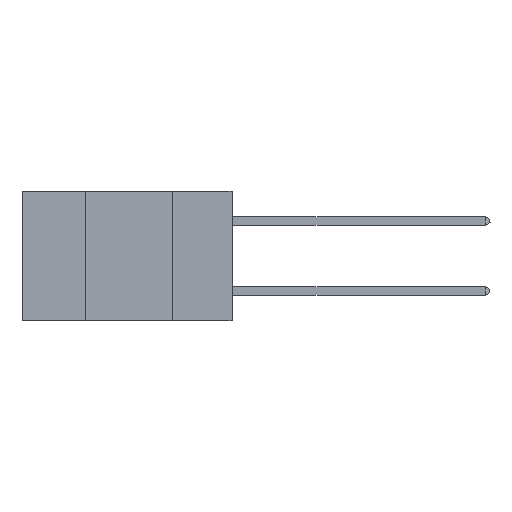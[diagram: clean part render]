
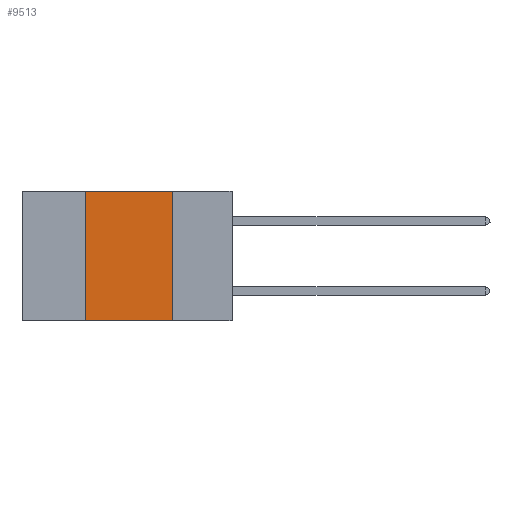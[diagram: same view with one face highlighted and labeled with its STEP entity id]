
A CAD part, left-side view. The second image highlights one B-rep face of the part: STEP entity #9513.
In plain terms, the highlighted planar face has unit normal (-1, 0, 0).
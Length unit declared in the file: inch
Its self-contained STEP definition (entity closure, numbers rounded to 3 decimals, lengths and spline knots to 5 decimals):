
#677 = FACE_OUTER_BOUND ( 'NONE', #10538, .T. ) ;
#836 = CARTESIAN_POINT ( 'NONE',  ( 0., 0.6, 0. ) ) ;
#1357 = DIRECTION ( 'NONE',  ( 0., 0., -1. ) ) ;
#1505 = CARTESIAN_POINT ( 'NONE',  ( 0., 0.17, 0. ) ) ;
#2086 = DIRECTION ( 'NONE',  ( 0., 0., -1. ) ) ;
#2443 = ORIENTED_EDGE ( 'NONE', *, *, #13610, .T. ) ;
#2631 = VERTEX_POINT ( 'NONE', #2935 ) ;
#2935 = CARTESIAN_POINT ( 'NONE',  ( 0., 0.42, -0.37 ) ) ;
#3378 = EDGE_CURVE ( 'NONE', #2631, #10087, #14278, .T. ) ;
#3678 = CARTESIAN_POINT ( 'NONE',  ( 0., 0.42, 0. ) ) ;
#3721 = EDGE_CURVE ( 'NONE', #13696, #7649, #4877, .T. ) ;
#3918 = ORIENTED_EDGE ( 'NONE', *, *, #11808, .F. ) ;
#4377 = DIRECTION ( 'NONE',  ( 0., -1., 0. ) ) ;
#4877 = LINE ( 'NONE', #1505, #5730 ) ;
#5730 = VECTOR ( 'NONE', #1357, 39.37008 ) ;
#5772 = DIRECTION ( 'NONE',  ( 0., -1., 0. ) ) ;
#5870 = VECTOR ( 'NONE', #5772, 39.37008 ) ;
#6531 = ORIENTED_EDGE ( 'NONE', *, *, #3378, .F. ) ;
#7090 = CARTESIAN_POINT ( 'NONE',  ( 0., 0.42, 0. ) ) ;
#7649 = VERTEX_POINT ( 'NONE', #13264 ) ;
#8371 = CARTESIAN_POINT ( 'NONE',  ( 0., 0.17, 0. ) ) ;
#9112 = LINE ( 'NONE', #12818, #5870 ) ;
#9513 = ADVANCED_FACE ( 'NONE', ( #677 ), #10375, .F. ) ;
#10087 = VERTEX_POINT ( 'NONE', #7090 ) ;
#10251 = LINE ( 'NONE', #14981, #12803 ) ;
#10375 = PLANE ( 'NONE',  #13741 ) ;
#10538 = EDGE_LOOP ( 'NONE', ( #10762, #3918, #6531, #2443 ) ) ;
#10762 = ORIENTED_EDGE ( 'NONE', *, *, #3721, .F. ) ;
#11808 = EDGE_CURVE ( 'NONE', #10087, #13696, #9112, .T. ) ;
#12803 = VECTOR ( 'NONE', #4377, 39.37008 ) ;
#12818 = CARTESIAN_POINT ( 'NONE',  ( 0., 0.6, 0. ) ) ;
#13118 = DIRECTION ( 'NONE',  ( 0., 0., 1. ) ) ;
#13264 = CARTESIAN_POINT ( 'NONE',  ( 0., 0.17, -0.37 ) ) ;
#13610 = EDGE_CURVE ( 'NONE', #2631, #7649, #10251, .T. ) ;
#13696 = VERTEX_POINT ( 'NONE', #8371 ) ;
#13741 = AXIS2_PLACEMENT_3D ( 'NONE', #836, #15177, #2086 ) ;
#14278 = LINE ( 'NONE', #3678, #14620 ) ;
#14620 = VECTOR ( 'NONE', #13118, 39.37008 ) ;
#14981 = CARTESIAN_POINT ( 'NONE',  ( 0., 0.6, -0.37 ) ) ;
#15177 = DIRECTION ( 'NONE',  ( 1., 0., 0. ) ) ;
